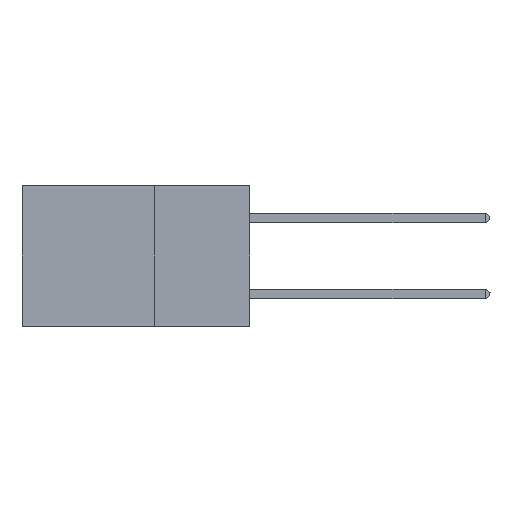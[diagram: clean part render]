
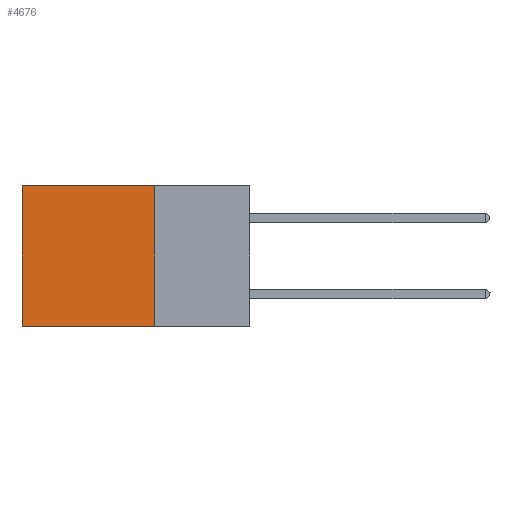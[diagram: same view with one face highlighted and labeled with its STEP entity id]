
A CAD part, left-side view. The second image highlights one B-rep face of the part: STEP entity #4676.
In plain terms, the highlighted planar face has unit normal (-1, 0, 0).
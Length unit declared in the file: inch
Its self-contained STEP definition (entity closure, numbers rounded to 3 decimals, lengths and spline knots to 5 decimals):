
#166 = FACE_OUTER_BOUND ( 'NONE', #14245, .T. ) ;
#424 = CARTESIAN_POINT ( 'NONE',  ( 0.2875, 0.25, 0. ) ) ;
#2356 = DIRECTION ( 'NONE',  ( 0., 1., 0. ) ) ;
#2364 = ORIENTED_EDGE ( 'NONE', *, *, #8473, .F. ) ;
#2412 = ORIENTED_EDGE ( 'NONE', *, *, #13008, .T. ) ;
#2442 = CARTESIAN_POINT ( 'NONE',  ( 0.2875, 0.25, -0.37 ) ) ;
#2955 = CARTESIAN_POINT ( 'NONE',  ( 0.2875, 0.6, 0. ) ) ;
#4425 = EDGE_CURVE ( 'NONE', #8117, #13942, #18719, .T. ) ;
#4676 = ADVANCED_FACE ( 'NONE', ( #166 ), #11734, .F. ) ;
#5061 = VECTOR ( 'NONE', #5850, 39.37008 ) ;
#5850 = DIRECTION ( 'NONE',  ( 0., 0., -1. ) ) ;
#8117 = VERTEX_POINT ( 'NONE', #20176 ) ;
#8275 = DIRECTION ( 'NONE',  ( 0., 0., -1. ) ) ;
#8473 = EDGE_CURVE ( 'NONE', #19443, #8117, #20218, .T. ) ;
#8840 = VERTEX_POINT ( 'NONE', #2955 ) ;
#9540 = VECTOR ( 'NONE', #8275, 39.37008 ) ;
#11690 = CARTESIAN_POINT ( 'NONE',  ( 0.2875, 0.6, -0.37 ) ) ;
#11734 = PLANE ( 'NONE',  #13546 ) ;
#11831 = ORIENTED_EDGE ( 'NONE', *, *, #4425, .F. ) ;
#11892 = EDGE_CURVE ( 'NONE', #19443, #8840, #14659, .T. ) ;
#13008 = EDGE_CURVE ( 'NONE', #8840, #13942, #14877, .T. ) ;
#13150 = DIRECTION ( 'NONE',  ( 0., 0., -1. ) ) ;
#13546 = AXIS2_PLACEMENT_3D ( 'NONE', #15725, #16597, #13150 ) ;
#13942 = VERTEX_POINT ( 'NONE', #11690 ) ;
#13958 = VECTOR ( 'NONE', #2356, 39.37008 ) ;
#14245 = EDGE_LOOP ( 'NONE', ( #2412, #11831, #2364, #22784 ) ) ;
#14659 = LINE ( 'NONE', #21553, #21386 ) ;
#14877 = LINE ( 'NONE', #22565, #9540 ) ;
#15725 = CARTESIAN_POINT ( 'NONE',  ( 0.2875, 0.25, 0. ) ) ;
#16597 = DIRECTION ( 'NONE',  ( 1., 0., 0. ) ) ;
#16621 = DIRECTION ( 'NONE',  ( 0., 1., 0. ) ) ;
#18719 = LINE ( 'NONE', #2442, #13958 ) ;
#19443 = VERTEX_POINT ( 'NONE', #20230 ) ;
#20176 = CARTESIAN_POINT ( 'NONE',  ( 0.2875, 0.25, -0.37 ) ) ;
#20218 = LINE ( 'NONE', #424, #5061 ) ;
#20230 = CARTESIAN_POINT ( 'NONE',  ( 0.2875, 0.25, 0. ) ) ;
#21386 = VECTOR ( 'NONE', #16621, 39.37008 ) ;
#21553 = CARTESIAN_POINT ( 'NONE',  ( 0.2875, 0.25, 0. ) ) ;
#22565 = CARTESIAN_POINT ( 'NONE',  ( 0.2875, 0.6, 0. ) ) ;
#22784 = ORIENTED_EDGE ( 'NONE', *, *, #11892, .T. ) ;
